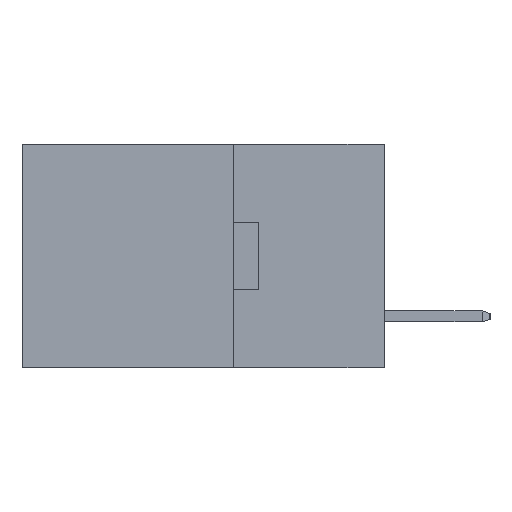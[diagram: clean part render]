
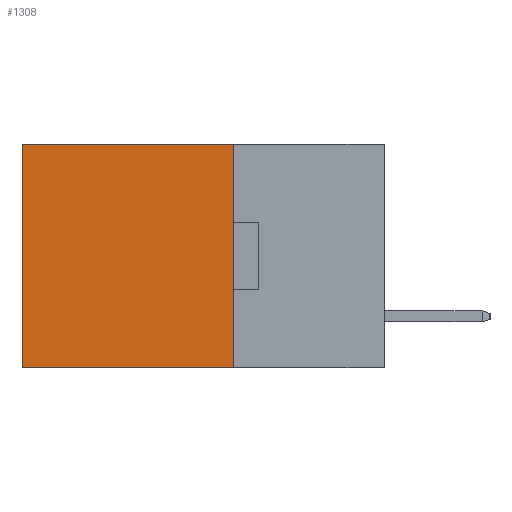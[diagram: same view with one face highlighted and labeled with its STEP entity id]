
A CAD part, left-side view. The second image highlights one B-rep face of the part: STEP entity #1308.
In plain terms, the highlighted planar face has unit normal (-1, 0, 0).
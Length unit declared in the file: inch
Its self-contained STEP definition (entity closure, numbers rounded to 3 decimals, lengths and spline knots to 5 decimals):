
#188 = CARTESIAN_POINT ( 'NONE',  ( 0.2615, 0.6, -0.37 ) ) ;
#320 = ORIENTED_EDGE ( 'NONE', *, *, #22436, .T. ) ;
#541 = VECTOR ( 'NONE', #8406, 39.37008 ) ;
#1194 = LINE ( 'NONE', #188, #541 ) ;
#1308 = ADVANCED_FACE ( 'NONE', ( #7707 ), #14727, .F. ) ;
#1523 = EDGE_CURVE ( 'NONE', #20575, #2007, #3162, .T. ) ;
#1866 = ORIENTED_EDGE ( 'NONE', *, *, #1523, .F. ) ;
#2007 = VERTEX_POINT ( 'NONE', #22812 ) ;
#2929 = ORIENTED_EDGE ( 'NONE', *, *, #8711, .F. ) ;
#3162 = LINE ( 'NONE', #6466, #18449 ) ;
#5784 = DIRECTION ( 'NONE',  ( 0., 0., -1. ) ) ;
#6425 = LINE ( 'NONE', #8911, #22357 ) ;
#6466 = CARTESIAN_POINT ( 'NONE',  ( 0.2615, 0.25, -0.37 ) ) ;
#7707 = FACE_OUTER_BOUND ( 'NONE', #15519, .T. ) ;
#8108 = AXIS2_PLACEMENT_3D ( 'NONE', #15528, #14695, #14487 ) ;
#8406 = DIRECTION ( 'NONE',  ( 0., 0., -1. ) ) ;
#8711 = EDGE_CURVE ( 'NONE', #2007, #14010, #26717, .T. ) ;
#8911 = CARTESIAN_POINT ( 'NONE',  ( 0.2615, 0.25, 0. ) ) ;
#9440 = VECTOR ( 'NONE', #22384, 39.37008 ) ;
#9851 = CARTESIAN_POINT ( 'NONE',  ( 0.2615, 0.25, -0.37 ) ) ;
#14010 = VERTEX_POINT ( 'NONE', #15110 ) ;
#14487 = DIRECTION ( 'NONE',  ( 0., 0., -1. ) ) ;
#14630 = CARTESIAN_POINT ( 'NONE',  ( 0.2615, 0.6, 0. ) ) ;
#14695 = DIRECTION ( 'NONE',  ( 1., 0., 0. ) ) ;
#14727 = PLANE ( 'NONE',  #8108 ) ;
#15110 = CARTESIAN_POINT ( 'NONE',  ( 0.2615, 0.6, -0.37 ) ) ;
#15178 = EDGE_CURVE ( 'NONE', #19701, #14010, #1194, .T. ) ;
#15519 = EDGE_LOOP ( 'NONE', ( #24303, #2929, #1866, #320 ) ) ;
#15528 = CARTESIAN_POINT ( 'NONE',  ( 0.2615, 0.25, -0.37 ) ) ;
#17190 = DIRECTION ( 'NONE',  ( 0., 1., 0. ) ) ;
#17396 = CARTESIAN_POINT ( 'NONE',  ( 0.2615, 0.25, 0. ) ) ;
#18449 = VECTOR ( 'NONE', #5784, 39.37008 ) ;
#19701 = VERTEX_POINT ( 'NONE', #14630 ) ;
#20575 = VERTEX_POINT ( 'NONE', #17396 ) ;
#22357 = VECTOR ( 'NONE', #17190, 39.37008 ) ;
#22384 = DIRECTION ( 'NONE',  ( 0., 1., 0. ) ) ;
#22436 = EDGE_CURVE ( 'NONE', #20575, #19701, #6425, .T. ) ;
#22812 = CARTESIAN_POINT ( 'NONE',  ( 0.2615, 0.25, -0.37 ) ) ;
#24303 = ORIENTED_EDGE ( 'NONE', *, *, #15178, .T. ) ;
#26717 = LINE ( 'NONE', #9851, #9440 ) ;
